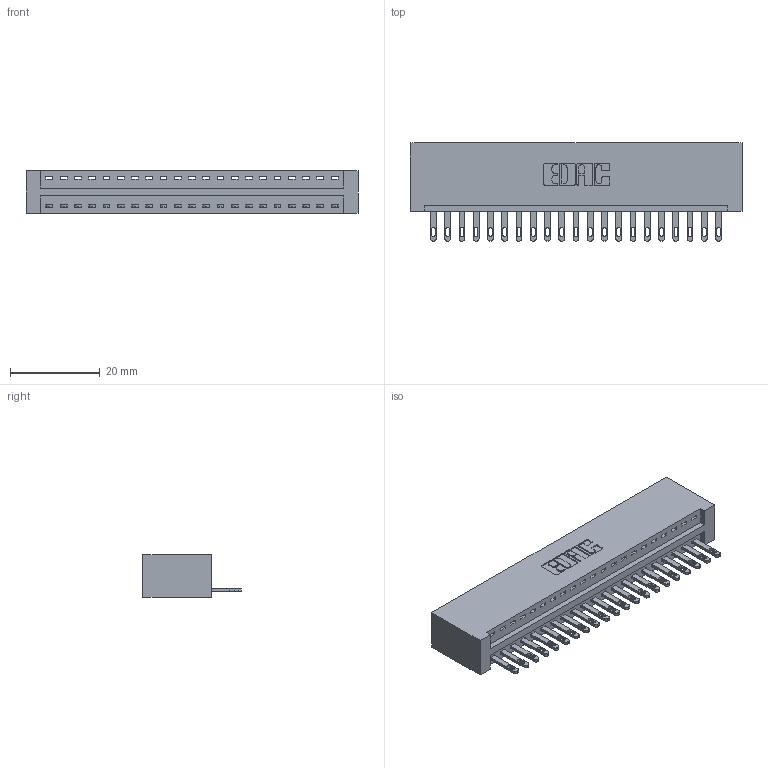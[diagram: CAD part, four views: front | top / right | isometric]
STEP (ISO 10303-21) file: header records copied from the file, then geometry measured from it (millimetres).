
FILE_DESCRIPTION (( 'STEP AP203' ), '1' );
FILE_NAME ('896-021-500-101.STEP', '2021-07-27T16:43:13', ( '' ), ( '' ), 'SwSTEP 2.0', 'SolidWorks 2020', '' );
FILE_SCHEMA (( 'CONFIG_CONTROL_DESIGN' ));
Length unit declared in the file: inch
Products named in the file (3): 846 Part_No Mounting Lugs; 896-021-500-101; 345-292-001_345-293-100
Assembly tree (22 placements, depth 2):
  896-021-500-101
    846 Part_No Mounting Lugs
    345-292-001_345-293-100  x21
Bounding box: 73.91 x 21.84 x 9.4 mm (x, y, z)
Volume: 7492.9 mm3; surface area: 9262.6 mm2
Topology: 22 solids, 22 shells, 1248 faces, 3833 edges, 2554 vertices
Faces by surface type: plane 786, cylinder 462
Entity records: 15513 total; most frequent: CARTESIAN_POINT 2671, ORIENTED_EDGE 2626, DIRECTION 2379, EDGE_CURVE 1313, VECTOR 1101, LINE 1101, VERTEX_POINT 874, AXIS2_PLACEMENT_3D 639
